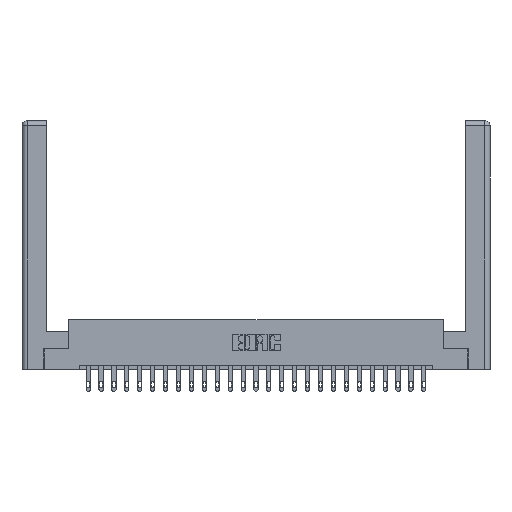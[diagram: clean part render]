
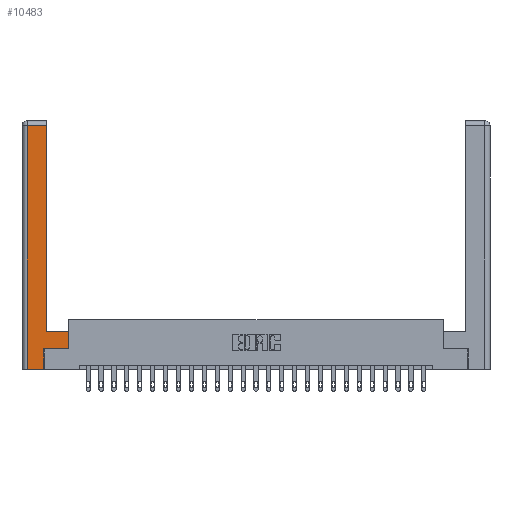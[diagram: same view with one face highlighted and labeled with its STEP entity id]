
A CAD part, top view. The second image highlights one B-rep face of the part: STEP entity #10483.
In plain terms, the highlighted planar face has unit normal (0, 0, 1).
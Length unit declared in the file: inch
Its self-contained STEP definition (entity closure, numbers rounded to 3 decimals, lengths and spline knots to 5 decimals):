
#209 = AXIS2_PLACEMENT_3D ( 'NONE', #974, #18752, #22438 ) ;
#304 = ORIENTED_EDGE ( 'NONE', *, *, #2325, .T. ) ;
#974 = CARTESIAN_POINT ( 'NONE',  ( 0., 0., 0. ) ) ;
#1189 = EDGE_CURVE ( 'NONE', #20347, #14077, #7701, .T. ) ;
#1319 = VECTOR ( 'NONE', #11337, 39.37008 ) ;
#1816 = DIRECTION ( 'NONE',  ( 0., 1., 0. ) ) ;
#2325 = EDGE_CURVE ( 'NONE', #9952, #22033, #11666, .T. ) ;
#2769 = VECTOR ( 'NONE', #21205, 39.37008 ) ;
#3427 = CARTESIAN_POINT ( 'NONE',  ( 0.565, 0.45, 0. ) ) ;
#3504 = EDGE_CURVE ( 'NONE', #22033, #18576, #10999, .T. ) ;
#3668 = VERTEX_POINT ( 'NONE', #14042 ) ;
#4498 = CARTESIAN_POINT ( 'NONE',  ( 0.565, 0.45, 0. ) ) ;
#5611 = EDGE_CURVE ( 'NONE', #18576, #14957, #22215, .T. ) ;
#5740 = VECTOR ( 'NONE', #9318, 39.37008 ) ;
#5928 = CARTESIAN_POINT ( 'NONE',  ( 0.265, 0., 0. ) ) ;
#6194 = ORIENTED_EDGE ( 'NONE', *, *, #21398, .T. ) ;
#6356 = VECTOR ( 'NONE', #23179, 39.37008 ) ;
#7292 = LINE ( 'NONE', #3427, #6356 ) ;
#7497 = CARTESIAN_POINT ( 'NONE',  ( 0.295, 3., 0. ) ) ;
#7583 = VECTOR ( 'NONE', #1816, 39.37008 ) ;
#7701 = LINE ( 'NONE', #25264, #2769 ) ;
#8539 = VECTOR ( 'NONE', #17644, 39.37008 ) ;
#8741 = EDGE_CURVE ( 'NONE', #3668, #9952, #7292, .T. ) ;
#9318 = DIRECTION ( 'NONE',  ( 0., 1., 0. ) ) ;
#9362 = CARTESIAN_POINT ( 'NONE',  ( 0.0615, 2.94, 0. ) ) ;
#9456 = EDGE_LOOP ( 'NONE', ( #12366, #17673, #16583, #22677, #6194, #9755, #11438, #304 ) ) ;
#9755 = ORIENTED_EDGE ( 'NONE', *, *, #13060, .T. ) ;
#9952 = VERTEX_POINT ( 'NONE', #4498 ) ;
#10483 = ADVANCED_FACE ( 'NONE', ( #21368 ), #24430, .F. ) ;
#10704 = CARTESIAN_POINT ( 'NONE',  ( 0.295, 2.94, 0. ) ) ;
#10940 = VERTEX_POINT ( 'NONE', #12324 ) ;
#10999 = LINE ( 'NONE', #7497, #5740 ) ;
#11337 = DIRECTION ( 'NONE',  ( -1., 0., 0. ) ) ;
#11438 = ORIENTED_EDGE ( 'NONE', *, *, #8741, .T. ) ;
#11666 = LINE ( 'NONE', #11808, #8539 ) ;
#11808 = CARTESIAN_POINT ( 'NONE',  ( 0.295, 0.45, 0. ) ) ;
#12324 = CARTESIAN_POINT ( 'NONE',  ( 0.265, 0.245, 0. ) ) ;
#12366 = ORIENTED_EDGE ( 'NONE', *, *, #3504, .T. ) ;
#13060 = EDGE_CURVE ( 'NONE', #10940, #3668, #13453, .T. ) ;
#13453 = LINE ( 'NONE', #24431, #16529 ) ;
#14042 = CARTESIAN_POINT ( 'NONE',  ( 0.565, 0.245, 0. ) ) ;
#14077 = VERTEX_POINT ( 'NONE', #5928 ) ;
#14458 = DIRECTION ( 'NONE',  ( 0., -1., 0. ) ) ;
#14957 = VERTEX_POINT ( 'NONE', #23896 ) ;
#15704 = CARTESIAN_POINT ( 'NONE',  ( 0.295, 0.45, 0. ) ) ;
#16529 = VECTOR ( 'NONE', #22699, 39.37008 ) ;
#16583 = ORIENTED_EDGE ( 'NONE', *, *, #18178, .T. ) ;
#17139 = VECTOR ( 'NONE', #14458, 39.37008 ) ;
#17644 = DIRECTION ( 'NONE',  ( -1., 0., 0. ) ) ;
#17673 = ORIENTED_EDGE ( 'NONE', *, *, #5611, .T. ) ;
#18042 = LINE ( 'NONE', #22943, #7583 ) ;
#18134 = CARTESIAN_POINT ( 'NONE',  ( 0.0615, 0., 0. ) ) ;
#18178 = EDGE_CURVE ( 'NONE', #14957, #20347, #19019, .T. ) ;
#18576 = VERTEX_POINT ( 'NONE', #10704 ) ;
#18752 = DIRECTION ( 'NONE',  ( 0., 0., -1. ) ) ;
#19019 = LINE ( 'NONE', #18134, #17139 ) ;
#20347 = VERTEX_POINT ( 'NONE', #25318 ) ;
#21205 = DIRECTION ( 'NONE',  ( 1., 0., 0. ) ) ;
#21368 = FACE_OUTER_BOUND ( 'NONE', #9456, .T. ) ;
#21398 = EDGE_CURVE ( 'NONE', #14077, #10940, #18042, .T. ) ;
#22033 = VERTEX_POINT ( 'NONE', #15704 ) ;
#22215 = LINE ( 'NONE', #9362, #1319 ) ;
#22438 = DIRECTION ( 'NONE',  ( -1., 0., 0. ) ) ;
#22677 = ORIENTED_EDGE ( 'NONE', *, *, #1189, .T. ) ;
#22699 = DIRECTION ( 'NONE',  ( 1., 0., 0. ) ) ;
#22943 = CARTESIAN_POINT ( 'NONE',  ( 0.265, 0.245, 0. ) ) ;
#23179 = DIRECTION ( 'NONE',  ( 0., 1., 0. ) ) ;
#23896 = CARTESIAN_POINT ( 'NONE',  ( 0.0615, 2.94, 0. ) ) ;
#24430 = PLANE ( 'NONE',  #209 ) ;
#24431 = CARTESIAN_POINT ( 'NONE',  ( 0.565, 0.245, 0. ) ) ;
#25264 = CARTESIAN_POINT ( 'NONE',  ( 0.265, 0., 0. ) ) ;
#25318 = CARTESIAN_POINT ( 'NONE',  ( 0.0615, 0., 0. ) ) ;
